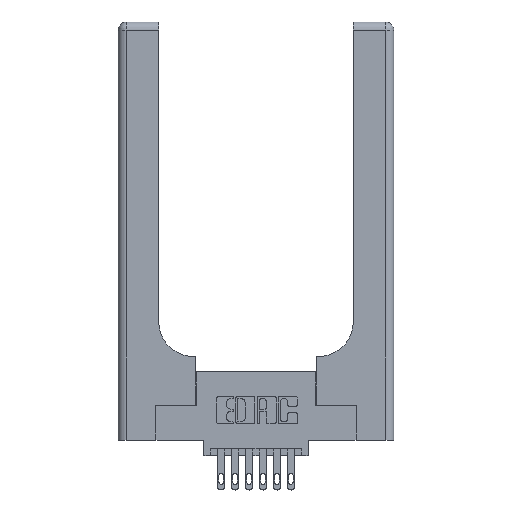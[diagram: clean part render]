
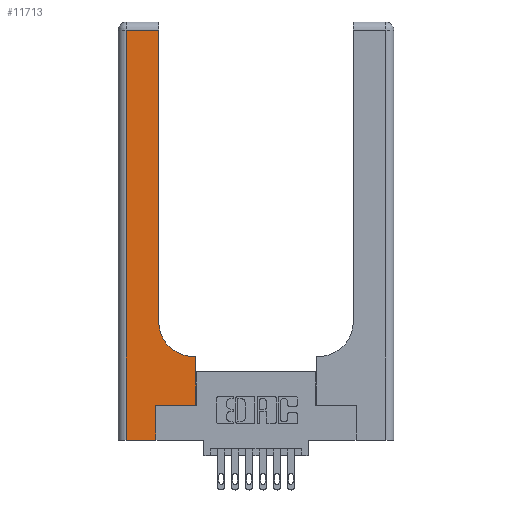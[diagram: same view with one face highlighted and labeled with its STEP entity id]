
A CAD part, top view. The second image highlights one B-rep face of the part: STEP entity #11713.
In plain terms, the highlighted planar face has unit normal (0, 0, 1).
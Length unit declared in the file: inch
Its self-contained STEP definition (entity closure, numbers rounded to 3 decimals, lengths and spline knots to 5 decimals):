
#143 = CARTESIAN_POINT ( 'NONE',  ( 0.2915, 3., 0.37 ) ) ;
#198 = DIRECTION ( 'NONE',  ( 0., -1., 0. ) ) ;
#285 = DIRECTION ( 'NONE',  ( 1., 0., 0. ) ) ;
#288 = LINE ( 'NONE', #12015, #3888 ) ;
#305 = CARTESIAN_POINT ( 'NONE',  ( 0.2915, 0.85, 0.37 ) ) ;
#829 = LINE ( 'NONE', #10304, #9628 ) ;
#1397 = PLANE ( 'NONE',  #13910 ) ;
#1442 = ORIENTED_EDGE ( 'NONE', *, *, #11586, .T. ) ;
#1503 = VERTEX_POINT ( 'NONE', #12894 ) ;
#2315 = ORIENTED_EDGE ( 'NONE', *, *, #5478, .T. ) ;
#3010 = CARTESIAN_POINT ( 'NONE',  ( 0.5415, 0.85, 0.37 ) ) ;
#3148 = CARTESIAN_POINT ( 'NONE',  ( 0.06, 2.94, 0.37 ) ) ;
#3168 = CIRCLE ( 'NONE', #14607, 0.25 ) ;
#3205 = VECTOR ( 'NONE', #7529, 39.37008 ) ;
#3243 = DIRECTION ( 'NONE',  ( 0., 1., 0. ) ) ;
#3494 = VERTEX_POINT ( 'NONE', #3909 ) ;
#3568 = CARTESIAN_POINT ( 'NONE',  ( 0.06, 3., 0.37 ) ) ;
#3613 = LINE ( 'NONE', #3568, #8267 ) ;
#3858 = VECTOR ( 'NONE', #3243, 39.37008 ) ;
#3888 = VECTOR ( 'NONE', #13966, 39.37008 ) ;
#3909 = CARTESIAN_POINT ( 'NONE',  ( 0.5585, 0.6, 0.37 ) ) ;
#4068 = VECTOR ( 'NONE', #11479, 39.37008 ) ;
#4143 = CARTESIAN_POINT ( 'NONE',  ( 0., 2.94, 0.37 ) ) ;
#4620 = VECTOR ( 'NONE', #12913, 39.37008 ) ;
#4669 = LINE ( 'NONE', #12807, #13432 ) ;
#4873 = CARTESIAN_POINT ( 'NONE',  ( 0.269, 0., 0.37 ) ) ;
#4875 = EDGE_CURVE ( 'NONE', #11079, #8451, #288, .T. ) ;
#4960 = VERTEX_POINT ( 'NONE', #13916 ) ;
#5144 = DIRECTION ( 'NONE',  ( 0., 0., -1. ) ) ;
#5236 = DIRECTION ( 'NONE',  ( 1., 0., 0. ) ) ;
#5376 = EDGE_CURVE ( 'NONE', #10669, #11079, #9610, .T. ) ;
#5439 = EDGE_CURVE ( 'NONE', #1503, #13509, #3168, .T. ) ;
#5478 = EDGE_CURVE ( 'NONE', #3494, #1503, #829, .T. ) ;
#5968 = VERTEX_POINT ( 'NONE', #3148 ) ;
#6281 = ORIENTED_EDGE ( 'NONE', *, *, #4875, .T. ) ;
#6431 = ORIENTED_EDGE ( 'NONE', *, *, #13873, .T. ) ;
#6477 = CARTESIAN_POINT ( 'NONE',  ( 0.06, 0., 0.37 ) ) ;
#6525 = EDGE_CURVE ( 'NONE', #4960, #3494, #6896, .T. ) ;
#6850 = ORIENTED_EDGE ( 'NONE', *, *, #6525, .T. ) ;
#6896 = LINE ( 'NONE', #12357, #3858 ) ;
#7321 = LINE ( 'NONE', #4143, #3205 ) ;
#7529 = DIRECTION ( 'NONE',  ( -1., 0., 0. ) ) ;
#7776 = VERTEX_POINT ( 'NONE', #9712 ) ;
#8006 = LINE ( 'NONE', #143, #4068 ) ;
#8267 = VECTOR ( 'NONE', #198, 39.37008 ) ;
#8362 = DIRECTION ( 'NONE',  ( 0., 0., -1. ) ) ;
#8451 = VERTEX_POINT ( 'NONE', #10806 ) ;
#9242 = EDGE_CURVE ( 'NONE', #5968, #10669, #3613, .T. ) ;
#9564 = CARTESIAN_POINT ( 'NONE',  ( 0., 3., 0.37 ) ) ;
#9610 = LINE ( 'NONE', #10672, #4620 ) ;
#9628 = VECTOR ( 'NONE', #11547, 39.37008 ) ;
#9712 = CARTESIAN_POINT ( 'NONE',  ( 0.2915, 2.94, 0.37 ) ) ;
#10127 = ORIENTED_EDGE ( 'NONE', *, *, #9242, .T. ) ;
#10304 = CARTESIAN_POINT ( 'NONE',  ( 0.2915, 0.6, 0.37 ) ) ;
#10518 = EDGE_LOOP ( 'NONE', ( #1442, #14787, #10127, #12462, #6281, #6431, #6850, #2315, #14741 ) ) ;
#10669 = VERTEX_POINT ( 'NONE', #6477 ) ;
#10672 = CARTESIAN_POINT ( 'NONE',  ( 0., 0., 0.37 ) ) ;
#10806 = CARTESIAN_POINT ( 'NONE',  ( 0.269, 0.25, 0.37 ) ) ;
#11079 = VERTEX_POINT ( 'NONE', #4873 ) ;
#11479 = DIRECTION ( 'NONE',  ( 0., 1., 0. ) ) ;
#11547 = DIRECTION ( 'NONE',  ( -1., 0., 0. ) ) ;
#11586 = EDGE_CURVE ( 'NONE', #13509, #7776, #8006, .T. ) ;
#11713 = ADVANCED_FACE ( 'NONE', ( #12489 ), #1397, .F. ) ;
#11869 = DIRECTION ( 'NONE',  ( -1., 0., 0. ) ) ;
#12015 = CARTESIAN_POINT ( 'NONE',  ( 0.269, 0., 0.37 ) ) ;
#12357 = CARTESIAN_POINT ( 'NONE',  ( 0.5585, 0.25, 0.37 ) ) ;
#12462 = ORIENTED_EDGE ( 'NONE', *, *, #5376, .T. ) ;
#12489 = FACE_OUTER_BOUND ( 'NONE', #10518, .T. ) ;
#12807 = CARTESIAN_POINT ( 'NONE',  ( 0.269, 0.25, 0.37 ) ) ;
#12894 = CARTESIAN_POINT ( 'NONE',  ( 0.5415, 0.6, 0.37 ) ) ;
#12913 = DIRECTION ( 'NONE',  ( 1., 0., 0. ) ) ;
#13432 = VECTOR ( 'NONE', #285, 39.37008 ) ;
#13509 = VERTEX_POINT ( 'NONE', #305 ) ;
#13873 = EDGE_CURVE ( 'NONE', #8451, #4960, #4669, .T. ) ;
#13910 = AXIS2_PLACEMENT_3D ( 'NONE', #9564, #8362, #11869 ) ;
#13916 = CARTESIAN_POINT ( 'NONE',  ( 0.5585, 0.25, 0.37 ) ) ;
#13966 = DIRECTION ( 'NONE',  ( 0., 1., 0. ) ) ;
#14105 = EDGE_CURVE ( 'NONE', #7776, #5968, #7321, .T. ) ;
#14607 = AXIS2_PLACEMENT_3D ( 'NONE', #3010, #5144, #5236 ) ;
#14741 = ORIENTED_EDGE ( 'NONE', *, *, #5439, .T. ) ;
#14787 = ORIENTED_EDGE ( 'NONE', *, *, #14105, .T. ) ;
